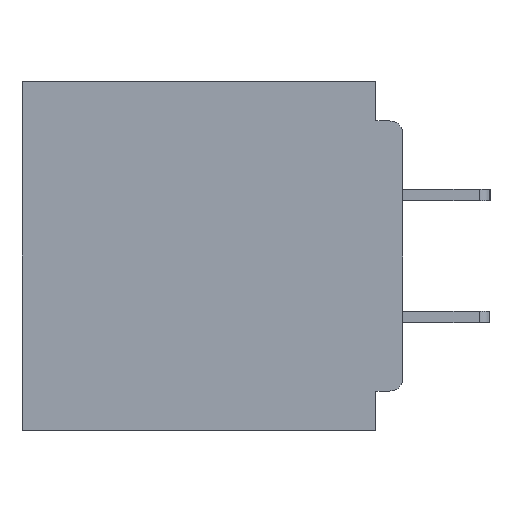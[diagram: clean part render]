
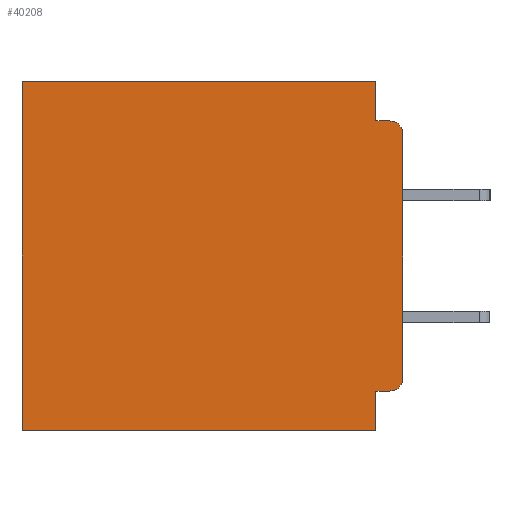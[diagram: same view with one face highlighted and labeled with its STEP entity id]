
A CAD part, left-side view. The second image highlights one B-rep face of the part: STEP entity #40208.
In plain terms, the highlighted planar face has unit normal (-1, 0, 0).
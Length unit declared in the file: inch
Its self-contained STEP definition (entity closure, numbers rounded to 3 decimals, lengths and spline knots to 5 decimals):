
#435 = CARTESIAN_POINT ( 'NONE',  ( 0.3, 0.015, -0.355 ) ) ;
#1482 = VECTOR ( 'NONE', #40544, 39.37008 ) ;
#2769 = LINE ( 'NONE', #31650, #46039 ) ;
#2872 = VERTEX_POINT ( 'NONE', #52759 ) ;
#2892 = ORIENTED_EDGE ( 'NONE', *, *, #12722, .F. ) ;
#3023 = CARTESIAN_POINT ( 'NONE',  ( 0.3, 0.031, -0.4 ) ) ;
#3126 = VERTEX_POINT ( 'NONE', #41745 ) ;
#3690 = AXIS2_PLACEMENT_3D ( 'NONE', #21242, #51312, #25586 ) ;
#4471 = DIRECTION ( 'NONE',  ( 1., 0., 0. ) ) ;
#5597 = AXIS2_PLACEMENT_3D ( 'NONE', #25282, #55311, #29653 ) ;
#6387 = VERTEX_POINT ( 'NONE', #53510 ) ;
#7370 = DIRECTION ( 'NONE',  ( 0., 0., -1. ) ) ;
#7832 = VERTEX_POINT ( 'NONE', #8681 ) ;
#8577 = CARTESIAN_POINT ( 'NONE',  ( 0.3, 0.437, 0. ) ) ;
#8681 = CARTESIAN_POINT ( 'NONE',  ( 0.3, 0.031, -0.4 ) ) ;
#9177 = CARTESIAN_POINT ( 'NONE',  ( 0.3, 0.031, 0. ) ) ;
#10024 = DIRECTION ( 'NONE',  ( 0., 0., -1. ) ) ;
#11815 = EDGE_CURVE ( 'NONE', #53410, #6387, #27068, .T. ) ;
#12630 = DIRECTION ( 'NONE',  ( 0., 0., -1. ) ) ;
#12722 = EDGE_CURVE ( 'NONE', #2872, #7832, #26970, .T. ) ;
#13562 = DIRECTION ( 'NONE',  ( 0., 0., -1. ) ) ;
#15738 = FACE_OUTER_BOUND ( 'NONE', #49708, .T. ) ;
#15979 = EDGE_CURVE ( 'NONE', #18617, #3126, #55444, .T. ) ;
#18617 = VERTEX_POINT ( 'NONE', #18818 ) ;
#18818 = CARTESIAN_POINT ( 'NONE',  ( 0.3, 0., -0.06 ) ) ;
#21242 = CARTESIAN_POINT ( 'NONE',  ( 0.3, 0.015, -0.34 ) ) ;
#21846 = VERTEX_POINT ( 'NONE', #52531 ) ;
#22549 = ORIENTED_EDGE ( 'NONE', *, *, #28787, .T. ) ;
#22717 = VECTOR ( 'NONE', #28986, 39.37008 ) ;
#23508 = ORIENTED_EDGE ( 'NONE', *, *, #51408, .F. ) ;
#23844 = DIRECTION ( 'NONE',  ( 0., 1., 0. ) ) ;
#24746 = CIRCLE ( 'NONE', #3690, 0.015 ) ;
#25282 = CARTESIAN_POINT ( 'NONE',  ( 0.3, 0.015, -0.06 ) ) ;
#25586 = DIRECTION ( 'NONE',  ( 0., 0., -1. ) ) ;
#25736 = VERTEX_POINT ( 'NONE', #36315 ) ;
#25909 = AXIS2_PLACEMENT_3D ( 'NONE', #30453, #4471, #34794 ) ;
#25921 = ORIENTED_EDGE ( 'NONE', *, *, #42310, .F. ) ;
#26970 = LINE ( 'NONE', #3023, #35747 ) ;
#27068 = LINE ( 'NONE', #9177, #48571 ) ;
#27160 = VECTOR ( 'NONE', #23844, 39.37008 ) ;
#28787 = EDGE_CURVE ( 'NONE', #46447, #25736, #2769, .T. ) ;
#28799 = ORIENTED_EDGE ( 'NONE', *, *, #51115, .T. ) ;
#28924 = ORIENTED_EDGE ( 'NONE', *, *, #11815, .F. ) ;
#28986 = DIRECTION ( 'NONE',  ( 0., 1., 0. ) ) ;
#29336 = ORIENTED_EDGE ( 'NONE', *, *, #44547, .F. ) ;
#29653 = DIRECTION ( 'NONE',  ( 0., 0., -1. ) ) ;
#30453 = CARTESIAN_POINT ( 'NONE',  ( 0.3, 0., -0.4 ) ) ;
#31650 = CARTESIAN_POINT ( 'NONE',  ( 0.3, 0.437, -0.4 ) ) ;
#31771 = LINE ( 'NONE', #32537, #33124 ) ;
#32537 = CARTESIAN_POINT ( 'NONE',  ( 0.3, 0., -0.355 ) ) ;
#32580 = EDGE_CURVE ( 'NONE', #42157, #21846, #24746, .T. ) ;
#32960 = CARTESIAN_POINT ( 'NONE',  ( 0.3, 0.031, 0. ) ) ;
#33073 = ORIENTED_EDGE ( 'NONE', *, *, #53466, .F. ) ;
#33124 = VECTOR ( 'NONE', #53867, 39.37008 ) ;
#33334 = CARTESIAN_POINT ( 'NONE',  ( 0.3, 0., -0.4 ) ) ;
#34710 = ORIENTED_EDGE ( 'NONE', *, *, #32580, .T. ) ;
#34794 = DIRECTION ( 'NONE',  ( 0., 0., -1. ) ) ;
#35747 = VECTOR ( 'NONE', #7370, 39.37008 ) ;
#36315 = CARTESIAN_POINT ( 'NONE',  ( 0.3, 0.437, -0.4 ) ) ;
#38606 = LINE ( 'NONE', #49622, #27160 ) ;
#40208 = ADVANCED_FACE ( 'NONE', ( #15738 ), #47525, .F. ) ;
#40544 = DIRECTION ( 'NONE',  ( 0., -1., 0. ) ) ;
#41745 = CARTESIAN_POINT ( 'NONE',  ( 0.3, 0.015, -0.045 ) ) ;
#42157 = VERTEX_POINT ( 'NONE', #435 ) ;
#42310 = EDGE_CURVE ( 'NONE', #6387, #3126, #47468, .T. ) ;
#42587 = VECTOR ( 'NONE', #12630, 39.37008 ) ;
#42837 = CARTESIAN_POINT ( 'NONE',  ( 0.3, 0., -0.4 ) ) ;
#44547 = EDGE_CURVE ( 'NONE', #42157, #2872, #31771, .T. ) ;
#45254 = LINE ( 'NONE', #42837, #42587 ) ;
#45613 = LINE ( 'NONE', #33334, #22717 ) ;
#46039 = VECTOR ( 'NONE', #10024, 39.37008 ) ;
#46447 = VERTEX_POINT ( 'NONE', #8577 ) ;
#47468 = LINE ( 'NONE', #48982, #1482 ) ;
#47525 = PLANE ( 'NONE',  #25909 ) ;
#48571 = VECTOR ( 'NONE', #13562, 39.37008 ) ;
#48982 = CARTESIAN_POINT ( 'NONE',  ( 0.3, 0., -0.045 ) ) ;
#49622 = CARTESIAN_POINT ( 'NONE',  ( 0.3, 0., 0. ) ) ;
#49708 = EDGE_LOOP ( 'NONE', ( #23508, #54364, #25921, #28924, #28799, #22549, #33073, #2892, #29336, #34710 ) ) ;
#51115 = EDGE_CURVE ( 'NONE', #53410, #46447, #38606, .T. ) ;
#51312 = DIRECTION ( 'NONE',  ( -1., 0., 0. ) ) ;
#51408 = EDGE_CURVE ( 'NONE', #18617, #21846, #45254, .T. ) ;
#52531 = CARTESIAN_POINT ( 'NONE',  ( 0.3, 0., -0.34 ) ) ;
#52759 = CARTESIAN_POINT ( 'NONE',  ( 0.3, 0.031, -0.355 ) ) ;
#53410 = VERTEX_POINT ( 'NONE', #32960 ) ;
#53466 = EDGE_CURVE ( 'NONE', #7832, #25736, #45613, .T. ) ;
#53510 = CARTESIAN_POINT ( 'NONE',  ( 0.3, 0.031, -0.045 ) ) ;
#53867 = DIRECTION ( 'NONE',  ( 0., 1., 0. ) ) ;
#54364 = ORIENTED_EDGE ( 'NONE', *, *, #15979, .T. ) ;
#55311 = DIRECTION ( 'NONE',  ( -1., 0., 0. ) ) ;
#55444 = CIRCLE ( 'NONE', #5597, 0.015 ) ;
